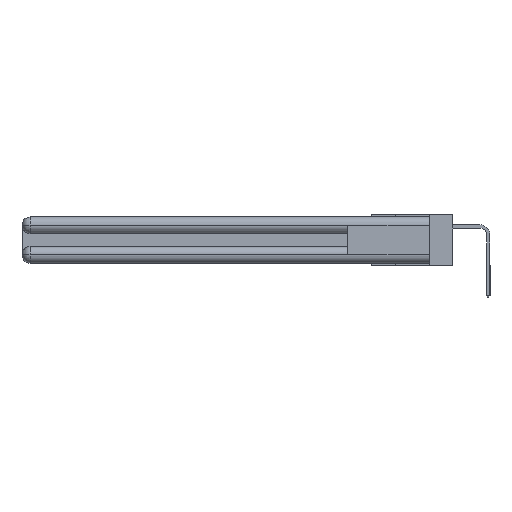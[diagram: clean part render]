
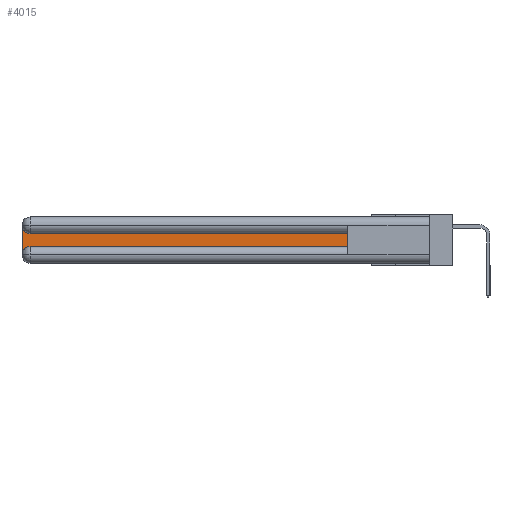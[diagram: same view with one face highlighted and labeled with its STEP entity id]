
A CAD part, left-side view. The second image highlights one B-rep face of the part: STEP entity #4015.
In plain terms, the highlighted planar face has unit normal (-1, 0, 0).
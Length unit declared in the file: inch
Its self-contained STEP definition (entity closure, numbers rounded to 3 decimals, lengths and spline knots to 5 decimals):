
#763 = DIRECTION ( 'NONE',  ( 0., 0., -1. ) ) ;
#878 = CARTESIAN_POINT ( 'NONE',  ( 0.075, 2.94, -0.0625 ) ) ;
#1463 = DIRECTION ( 'NONE',  ( 0., 1., 0. ) ) ;
#1705 = VERTEX_POINT ( 'NONE', #10819 ) ;
#2033 = ORIENTED_EDGE ( 'NONE', *, *, #3839, .T. ) ;
#2186 = VERTEX_POINT ( 'NONE', #27354 ) ;
#3499 = VERTEX_POINT ( 'NONE', #17856 ) ;
#3839 = EDGE_CURVE ( 'NONE', #1705, #2186, #5043, .T. ) ;
#3886 = AXIS2_PLACEMENT_3D ( 'NONE', #13955, #11425, #14166 ) ;
#4015 = ADVANCED_FACE ( 'NONE', ( #14149 ), #28575, .F. ) ;
#5043 = CIRCLE ( 'NONE', #27222, 0.06 ) ;
#5108 = LINE ( 'NONE', #11319, #15420 ) ;
#6308 = EDGE_CURVE ( 'NONE', #2186, #10710, #17831, .T. ) ;
#6366 = EDGE_LOOP ( 'NONE', ( #16810, #2033, #22557, #9294, #6446, #17750 ) ) ;
#6446 = ORIENTED_EDGE ( 'NONE', *, *, #9745, .T. ) ;
#9294 = ORIENTED_EDGE ( 'NONE', *, *, #22321, .T. ) ;
#9745 = EDGE_CURVE ( 'NONE', #24061, #15674, #5108, .T. ) ;
#9836 = VECTOR ( 'NONE', #1463, 39.37008 ) ;
#10710 = VERTEX_POINT ( 'NONE', #30365 ) ;
#10819 = CARTESIAN_POINT ( 'NONE',  ( 0.075, 2.94, -0.1225 ) ) ;
#11319 = CARTESIAN_POINT ( 'NONE',  ( 0.075, 0.6, -0.2175 ) ) ;
#11425 = DIRECTION ( 'NONE',  ( 1., 0., 0. ) ) ;
#12697 = DIRECTION ( 'NONE',  ( 1., 0., 0. ) ) ;
#12916 = DIRECTION ( 'NONE',  ( 0., 0., -1. ) ) ;
#12918 = DIRECTION ( 'NONE',  ( 0., 0., -1. ) ) ;
#13097 = CARTESIAN_POINT ( 'NONE',  ( 0.075, 0.6, -0.2175 ) ) ;
#13348 = CIRCLE ( 'NONE', #31466, 0.06 ) ;
#13955 = CARTESIAN_POINT ( 'NONE',  ( 0.075, 3., -0.1225 ) ) ;
#14149 = FACE_OUTER_BOUND ( 'NONE', #6366, .T. ) ;
#14166 = DIRECTION ( 'NONE',  ( 0., 0., -1. ) ) ;
#15420 = VECTOR ( 'NONE', #16044, 39.37008 ) ;
#15551 = VECTOR ( 'NONE', #12916, 39.37008 ) ;
#15674 = VERTEX_POINT ( 'NONE', #13097 ) ;
#15756 = DIRECTION ( 'NONE',  ( 1., 0., 0. ) ) ;
#16044 = DIRECTION ( 'NONE',  ( 0., -1., 0. ) ) ;
#16306 = LINE ( 'NONE', #25951, #9836 ) ;
#16810 = ORIENTED_EDGE ( 'NONE', *, *, #26144, .T. ) ;
#17750 = ORIENTED_EDGE ( 'NONE', *, *, #17902, .T. ) ;
#17831 = LINE ( 'NONE', #20276, #15551 ) ;
#17856 = CARTESIAN_POINT ( 'NONE',  ( 0.075, 0.6, -0.1225 ) ) ;
#17902 = EDGE_CURVE ( 'NONE', #15674, #3499, #24736, .T. ) ;
#20276 = CARTESIAN_POINT ( 'NONE',  ( 0.075, 3., -0.2175 ) ) ;
#20531 = VECTOR ( 'NONE', #28941, 39.37008 ) ;
#21729 = CARTESIAN_POINT ( 'NONE',  ( 0.075, 0.6, -0.2175 ) ) ;
#22321 = EDGE_CURVE ( 'NONE', #10710, #24061, #13348, .T. ) ;
#22557 = ORIENTED_EDGE ( 'NONE', *, *, #6308, .T. ) ;
#24061 = VERTEX_POINT ( 'NONE', #24180 ) ;
#24180 = CARTESIAN_POINT ( 'NONE',  ( 0.075, 2.94, -0.2175 ) ) ;
#24736 = LINE ( 'NONE', #21729, #20531 ) ;
#25109 = CARTESIAN_POINT ( 'NONE',  ( 0.075, 2.94, -0.2775 ) ) ;
#25951 = CARTESIAN_POINT ( 'NONE',  ( 0.075, 0.6, -0.1225 ) ) ;
#26144 = EDGE_CURVE ( 'NONE', #3499, #1705, #16306, .T. ) ;
#27222 = AXIS2_PLACEMENT_3D ( 'NONE', #878, #15756, #763 ) ;
#27354 = CARTESIAN_POINT ( 'NONE',  ( 0.075, 3., -0.0625 ) ) ;
#28575 = PLANE ( 'NONE',  #3886 ) ;
#28941 = DIRECTION ( 'NONE',  ( 0., 0., 1. ) ) ;
#30365 = CARTESIAN_POINT ( 'NONE',  ( 0.075, 3., -0.2775 ) ) ;
#31466 = AXIS2_PLACEMENT_3D ( 'NONE', #25109, #12697, #12918 ) ;
